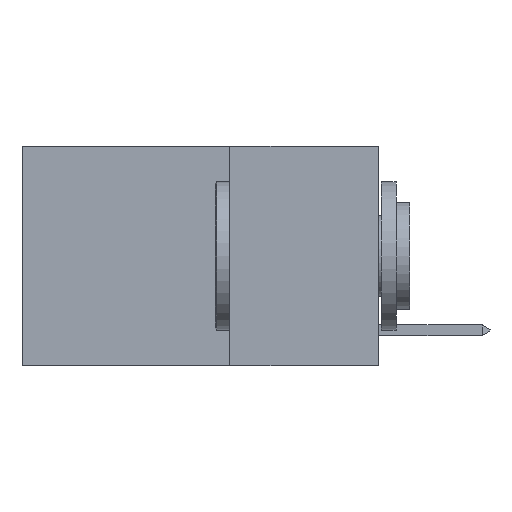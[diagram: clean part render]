
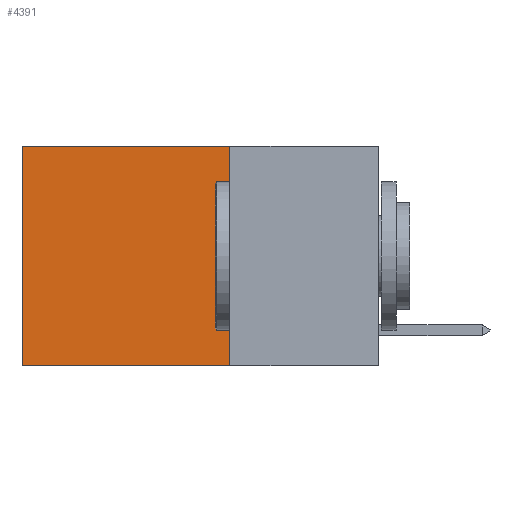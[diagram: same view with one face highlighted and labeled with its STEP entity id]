
A CAD part, left-side view. The second image highlights one B-rep face of the part: STEP entity #4391.
In plain terms, the highlighted planar face has unit normal (-1, 0, 0).
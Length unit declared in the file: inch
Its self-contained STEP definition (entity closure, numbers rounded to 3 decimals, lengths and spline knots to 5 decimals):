
#133 = DIRECTION ( 'NONE',  ( 0., 1., 0. ) ) ;
#224 = LINE ( 'NONE', #8711, #3540 ) ;
#272 = CARTESIAN_POINT ( 'NONE',  ( 0.2625, 0.6, -0.37 ) ) ;
#408 = ORIENTED_EDGE ( 'NONE', *, *, #1437, .F. ) ;
#594 = EDGE_CURVE ( 'NONE', #1508, #2204, #7974, .T. ) ;
#1011 = CARTESIAN_POINT ( 'NONE',  ( 0.2625, 0.25, -0.37 ) ) ;
#1437 = EDGE_CURVE ( 'NONE', #4408, #9145, #224, .T. ) ;
#1475 = ORIENTED_EDGE ( 'NONE', *, *, #2058, .F. ) ;
#1508 = VERTEX_POINT ( 'NONE', #7469 ) ;
#1760 = DIRECTION ( 'NONE',  ( 0., 0., -1. ) ) ;
#1912 = VECTOR ( 'NONE', #4544, 39.37008 ) ;
#2058 = EDGE_CURVE ( 'NONE', #9145, #2204, #5284, .T. ) ;
#2204 = VERTEX_POINT ( 'NONE', #272 ) ;
#2789 = DIRECTION ( 'NONE',  ( 0., 0., -1. ) ) ;
#3245 = EDGE_CURVE ( 'NONE', #4408, #1508, #6915, .T. ) ;
#3263 = CARTESIAN_POINT ( 'NONE',  ( 0.2625, 0.25, 0. ) ) ;
#3304 = DIRECTION ( 'NONE',  ( 1., 0., 0. ) ) ;
#3540 = VECTOR ( 'NONE', #2789, 39.37008 ) ;
#3835 = VECTOR ( 'NONE', #8729, 39.37008 ) ;
#4024 = CARTESIAN_POINT ( 'NONE',  ( 0.2625, 0.25, 0. ) ) ;
#4139 = ORIENTED_EDGE ( 'NONE', *, *, #3245, .T. ) ;
#4391 = ADVANCED_FACE ( 'NONE', ( #8684 ), #4817, .F. ) ;
#4408 = VERTEX_POINT ( 'NONE', #4024 ) ;
#4544 = DIRECTION ( 'NONE',  ( 0., 1., 0. ) ) ;
#4634 = VECTOR ( 'NONE', #133, 39.37008 ) ;
#4717 = EDGE_LOOP ( 'NONE', ( #6525, #1475, #408, #4139 ) ) ;
#4817 = PLANE ( 'NONE',  #8196 ) ;
#5284 = LINE ( 'NONE', #6873, #4634 ) ;
#6171 = CARTESIAN_POINT ( 'NONE',  ( 0.2625, 0.25, 0. ) ) ;
#6525 = ORIENTED_EDGE ( 'NONE', *, *, #594, .T. ) ;
#6873 = CARTESIAN_POINT ( 'NONE',  ( 0.2625, 0.25, -0.37 ) ) ;
#6915 = LINE ( 'NONE', #6171, #1912 ) ;
#7272 = CARTESIAN_POINT ( 'NONE',  ( 0.2625, 0.6, 0. ) ) ;
#7469 = CARTESIAN_POINT ( 'NONE',  ( 0.2625, 0.6, 0. ) ) ;
#7974 = LINE ( 'NONE', #7272, #3835 ) ;
#8196 = AXIS2_PLACEMENT_3D ( 'NONE', #3263, #3304, #1760 ) ;
#8684 = FACE_OUTER_BOUND ( 'NONE', #4717, .T. ) ;
#8711 = CARTESIAN_POINT ( 'NONE',  ( 0.2625, 0.25, 0. ) ) ;
#8729 = DIRECTION ( 'NONE',  ( 0., 0., -1. ) ) ;
#9145 = VERTEX_POINT ( 'NONE', #1011 ) ;
